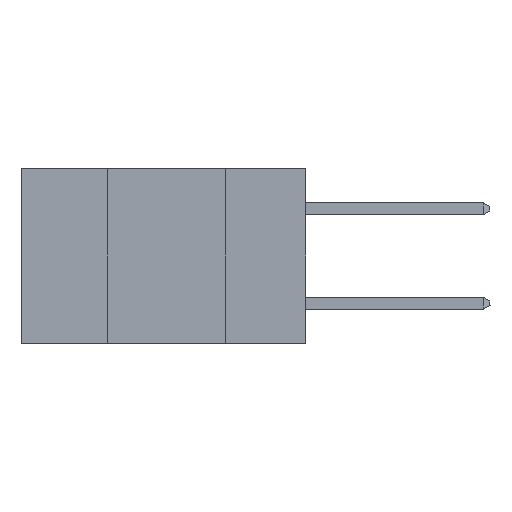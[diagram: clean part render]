
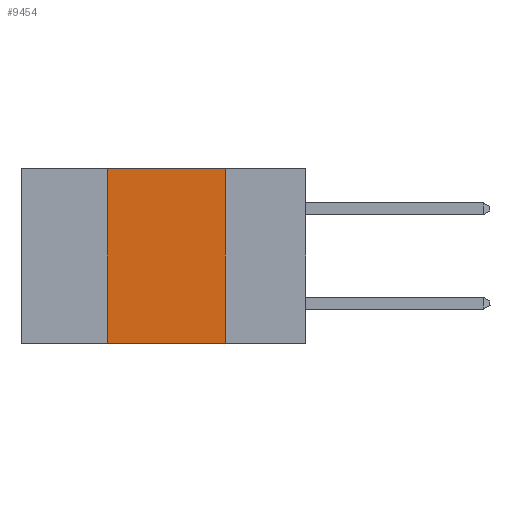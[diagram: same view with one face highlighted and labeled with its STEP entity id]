
A CAD part, left-side view. The second image highlights one B-rep face of the part: STEP entity #9454.
In plain terms, the highlighted planar face has unit normal (-1, 0, 0).
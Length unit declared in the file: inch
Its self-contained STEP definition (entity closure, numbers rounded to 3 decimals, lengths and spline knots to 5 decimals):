
#1404 = VERTEX_POINT ( 'NONE', #20792 ) ;
#2353 = LINE ( 'NONE', #7216, #12537 ) ;
#5269 = VECTOR ( 'NONE', #24538, 39.37008 ) ;
#5683 = VERTEX_POINT ( 'NONE', #24363 ) ;
#6002 = PLANE ( 'NONE',  #18915 ) ;
#6237 = LINE ( 'NONE', #19086, #19786 ) ;
#7216 = CARTESIAN_POINT ( 'NONE',  ( 0., 0.6, 0. ) ) ;
#7655 = DIRECTION ( 'NONE',  ( 0., -1., 0. ) ) ;
#7837 = VERTEX_POINT ( 'NONE', #23874 ) ;
#7979 = DIRECTION ( 'NONE',  ( 1., 0., 0. ) ) ;
#8469 = LINE ( 'NONE', #18261, #17506 ) ;
#8822 = VERTEX_POINT ( 'NONE', #15332 ) ;
#9161 = DIRECTION ( 'NONE',  ( 0., -1., 0. ) ) ;
#9454 = ADVANCED_FACE ( 'NONE', ( #18318 ), #6002, .F. ) ;
#10262 = ORIENTED_EDGE ( 'NONE', *, *, #11868, .F. ) ;
#10634 = ORIENTED_EDGE ( 'NONE', *, *, #17654, .T. ) ;
#11868 = EDGE_CURVE ( 'NONE', #7837, #1404, #2353, .T. ) ;
#12283 = LINE ( 'NONE', #22714, #5269 ) ;
#12537 = VECTOR ( 'NONE', #9161, 39.37008 ) ;
#15332 = CARTESIAN_POINT ( 'NONE',  ( 0., 0.17, -0.37 ) ) ;
#17506 = VECTOR ( 'NONE', #23934, 39.37008 ) ;
#17654 = EDGE_CURVE ( 'NONE', #5683, #8822, #6237, .T. ) ;
#18261 = CARTESIAN_POINT ( 'NONE',  ( 0., 0.42, 0. ) ) ;
#18318 = FACE_OUTER_BOUND ( 'NONE', #18671, .T. ) ;
#18671 = EDGE_LOOP ( 'NONE', ( #22643, #10262, #19881, #10634 ) ) ;
#18915 = AXIS2_PLACEMENT_3D ( 'NONE', #19479, #7979, #21367 ) ;
#18923 = EDGE_CURVE ( 'NONE', #1404, #8822, #12283, .T. ) ;
#19086 = CARTESIAN_POINT ( 'NONE',  ( 0., 0.6, -0.37 ) ) ;
#19479 = CARTESIAN_POINT ( 'NONE',  ( 0., 0.6, 0. ) ) ;
#19786 = VECTOR ( 'NONE', #7655, 39.37008 ) ;
#19881 = ORIENTED_EDGE ( 'NONE', *, *, #23953, .F. ) ;
#20792 = CARTESIAN_POINT ( 'NONE',  ( 0., 0.17, 0. ) ) ;
#21367 = DIRECTION ( 'NONE',  ( 0., 0., -1. ) ) ;
#22643 = ORIENTED_EDGE ( 'NONE', *, *, #18923, .F. ) ;
#22714 = CARTESIAN_POINT ( 'NONE',  ( 0., 0.17, 0. ) ) ;
#23874 = CARTESIAN_POINT ( 'NONE',  ( 0., 0.42, 0. ) ) ;
#23934 = DIRECTION ( 'NONE',  ( 0., 0., 1. ) ) ;
#23953 = EDGE_CURVE ( 'NONE', #5683, #7837, #8469, .T. ) ;
#24363 = CARTESIAN_POINT ( 'NONE',  ( 0., 0.42, -0.37 ) ) ;
#24538 = DIRECTION ( 'NONE',  ( 0., 0., -1. ) ) ;
